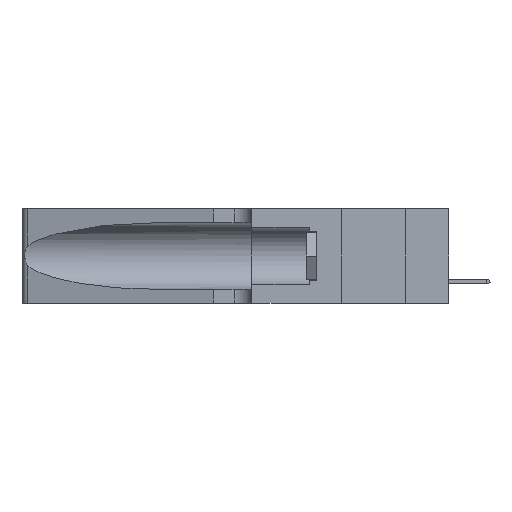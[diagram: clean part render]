
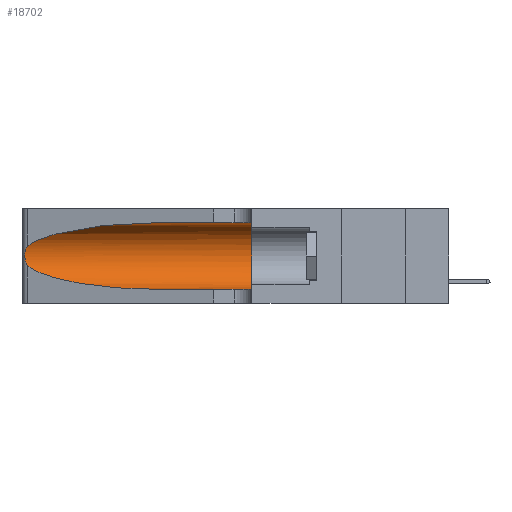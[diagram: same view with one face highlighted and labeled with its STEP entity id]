
A CAD part, left-side view. The second image highlights one B-rep face of the part: STEP entity #18702.
In plain terms, the highlighted cylindrical face has radius 3.308 mm (diameter 6.617 mm), a partial arc.
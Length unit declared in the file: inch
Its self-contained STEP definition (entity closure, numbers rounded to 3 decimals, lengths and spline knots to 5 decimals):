
#359 = CARTESIAN_POINT ( 'NONE',  ( 0.1305, 0.35, 0.31525 ) ) ;
#434 = DIRECTION ( 'NONE',  ( 0., 0., -1. ) ) ;
#682 = VERTEX_POINT ( 'NONE', #19937 ) ;
#683 = CARTESIAN_POINT ( 'NONE',  ( 0.1305, 1.61858, 0.185 ) ) ;
#1373 = CARTESIAN_POINT ( 'NONE',  ( 0.1305, 0.72297, 0.31525 ) ) ;
#1666 =( BOUNDED_CURVE ( )  B_SPLINE_CURVE ( 3, ( #12992, #32684, #1804, #12469 ),
 .UNSPECIFIED., .F., .F. ) 
 B_SPLINE_CURVE_WITH_KNOTS ( ( 4, 4 ),
 ( 3.44316, 4.71239 ),
 .UNSPECIFIED. ) 
 CURVE ( )  GEOMETRIC_REPRESENTATION_ITEM ( )  RATIONAL_B_SPLINE_CURVE ( ( 1., 0.87, 0.87, 1. ) ) 
 REPRESENTATION_ITEM ( '' )  );
#1767 = CARTESIAN_POINT ( 'NONE',  ( 0.25487, 1.22718, 0.22369 ) ) ;
#1804 = CARTESIAN_POINT ( 'NONE',  ( 0.18966, 0.96281, 0.05475 ) ) ;
#2543 = CARTESIAN_POINT ( 'NONE',  ( 0.26075, 1.23896, 0.178 ) ) ;
#2770 = CARTESIAN_POINT ( 'NONE',  ( 0.25639, 1.23186, 0.15144 ) ) ;
#5811 = VECTOR ( 'NONE', #33889, 39.37008 ) ;
#6346 = LINE ( 'NONE', #32205, #35445 ) ;
#6409 = ORIENTED_EDGE ( 'NONE', *, *, #29529, .F. ) ;
#6735 = DIRECTION ( 'NONE',  ( 0., 1., 0. ) ) ;
#6750 = CARTESIAN_POINT ( 'NONE',  ( 0.25487, 1.22718, 0.14631 ) ) ;
#7083 = EDGE_CURVE ( 'NONE', #20570, #682, #1666, .T. ) ;
#9509 = ORIENTED_EDGE ( 'NONE', *, *, #30566, .T. ) ;
#9782 = VERTEX_POINT ( 'NONE', #1767 ) ;
#9799 = AXIS2_PLACEMENT_3D ( 'NONE', #21064, #6735, #18229 ) ;
#9834 = FACE_OUTER_BOUND ( 'NONE', #36149, .T. ) ;
#11349 = CARTESIAN_POINT ( 'NONE',  ( 0.25487, 1.22718, 0.22369 ) ) ;
#11742 = ORIENTED_EDGE ( 'NONE', *, *, #35502, .F. ) ;
#12469 = CARTESIAN_POINT ( 'NONE',  ( 0.1305, 0.72297, 0.05475 ) ) ;
#12992 = CARTESIAN_POINT ( 'NONE',  ( 0.25487, 1.22718, 0.14631 ) ) ;
#13992 = CARTESIAN_POINT ( 'NONE',  ( 0.26075, 1.23896, 0.19203 ) ) ;
#15428 = EDGE_CURVE ( 'NONE', #29724, #9782, #26255, .T. ) ;
#16021 = CYLINDRICAL_SURFACE ( 'NONE', #26743, 0.13025 ) ;
#16708 = CARTESIAN_POINT ( 'NONE',  ( 0.26018, 1.23835, 0.19895 ) ) ;
#16816 = CARTESIAN_POINT ( 'NONE',  ( 0.1305, 0.35, 0.05475 ) ) ;
#17352 = DIRECTION ( 'NONE',  ( 0., -1., 0. ) ) ;
#17955 = DIRECTION ( 'NONE',  ( 0., -1., 0. ) ) ;
#18023 = CARTESIAN_POINT ( 'NONE',  ( 0.2373, 1.15595, 0.28018 ) ) ;
#18229 = DIRECTION ( 'NONE',  ( 0., 0., 1. ) ) ;
#18702 = ADVANCED_FACE ( 'NONE', ( #9834 ), #16021, .F. ) ;
#19671 = CARTESIAN_POINT ( 'NONE',  ( 0.25555, 1.22994, 0.2215 ) ) ;
#19892 = CARTESIAN_POINT ( 'NONE',  ( 0.25789, 1.23486, 0.15765 ) ) ;
#19928 = B_SPLINE_CURVE_WITH_KNOTS ( 'NONE', 3,
 ( #11349, #19671, #30634, #28031, #36234, #16708, #13992, #2543, #36470, #36344, #19892, #2770, #22237, #33785 ),
 .UNSPECIFIED., .F., .F.,
 ( 4, 2, 2, 2, 2, 2, 4 ),
 ( 0., 0.00027, 0.00053, 0.00107, 0.0016, 0.00187, 0.00214 ),
 .UNSPECIFIED. ) ;
#19937 = CARTESIAN_POINT ( 'NONE',  ( 0.1305, 0.72297, 0.05475 ) ) ;
#20273 = VERTEX_POINT ( 'NONE', #359 ) ;
#20403 = LINE ( 'NONE', #22583, #5811 ) ;
#20570 = VERTEX_POINT ( 'NONE', #6750 ) ;
#21064 = CARTESIAN_POINT ( 'NONE',  ( 0.1305, 0.35, 0.185 ) ) ;
#22237 = CARTESIAN_POINT ( 'NONE',  ( 0.25555, 1.22993, 0.14849 ) ) ;
#22432 = VERTEX_POINT ( 'NONE', #16816 ) ;
#22583 = CARTESIAN_POINT ( 'NONE',  ( 0.1305, 1.61858, 0.31525 ) ) ;
#24671 = ORIENTED_EDGE ( 'NONE', *, *, #15428, .T. ) ;
#24733 = CIRCLE ( 'NONE', #9799, 0.13025 ) ;
#24971 = ORIENTED_EDGE ( 'NONE', *, *, #25503, .T. ) ;
#25503 = EDGE_CURVE ( 'NONE', #682, #22432, #6346, .T. ) ;
#26255 =( BOUNDED_CURVE ( )  B_SPLINE_CURVE ( 3, ( #1373, #29595, #18023, #32030 ),
 .UNSPECIFIED., .F., .F. ) 
 B_SPLINE_CURVE_WITH_KNOTS ( ( 4, 4 ),
 ( 1.5708, 2.84003 ),
 .UNSPECIFIED. ) 
 CURVE ( )  GEOMETRIC_REPRESENTATION_ITEM ( )  RATIONAL_B_SPLINE_CURVE ( ( 1., 0.87, 0.87, 1. ) ) 
 REPRESENTATION_ITEM ( '' )  );
#26743 = AXIS2_PLACEMENT_3D ( 'NONE', #683, #17352, #434 ) ;
#28031 = CARTESIAN_POINT ( 'NONE',  ( 0.25787, 1.23484, 0.2124 ) ) ;
#29529 = EDGE_CURVE ( 'NONE', #20273, #22432, #24733, .T. ) ;
#29595 = CARTESIAN_POINT ( 'NONE',  ( 0.18966, 0.96281, 0.31525 ) ) ;
#29724 = VERTEX_POINT ( 'NONE', #35660 ) ;
#30499 = ORIENTED_EDGE ( 'NONE', *, *, #7083, .T. ) ;
#30566 = EDGE_CURVE ( 'NONE', #9782, #20570, #19928, .T. ) ;
#30634 = CARTESIAN_POINT ( 'NONE',  ( 0.25639, 1.23184, 0.21858 ) ) ;
#32030 = CARTESIAN_POINT ( 'NONE',  ( 0.25487, 1.22718, 0.22369 ) ) ;
#32205 = CARTESIAN_POINT ( 'NONE',  ( 0.1305, 1.61858, 0.05475 ) ) ;
#32684 = CARTESIAN_POINT ( 'NONE',  ( 0.2373, 1.15595, 0.08982 ) ) ;
#33785 = CARTESIAN_POINT ( 'NONE',  ( 0.25487, 1.22718, 0.14631 ) ) ;
#33889 = DIRECTION ( 'NONE',  ( 0., -1., 0. ) ) ;
#35445 = VECTOR ( 'NONE', #17955, 39.37008 ) ;
#35502 = EDGE_CURVE ( 'NONE', #29724, #20273, #20403, .T. ) ;
#35660 = CARTESIAN_POINT ( 'NONE',  ( 0.1305, 0.72297, 0.31525 ) ) ;
#36149 = EDGE_LOOP ( 'NONE', ( #24671, #9509, #30499, #24971, #6409, #11742 ) ) ;
#36234 = CARTESIAN_POINT ( 'NONE',  ( 0.25854, 1.2359, 0.20912 ) ) ;
#36344 = CARTESIAN_POINT ( 'NONE',  ( 0.25856, 1.23593, 0.16098 ) ) ;
#36470 = CARTESIAN_POINT ( 'NONE',  ( 0.26017, 1.23833, 0.17102 ) ) ;
